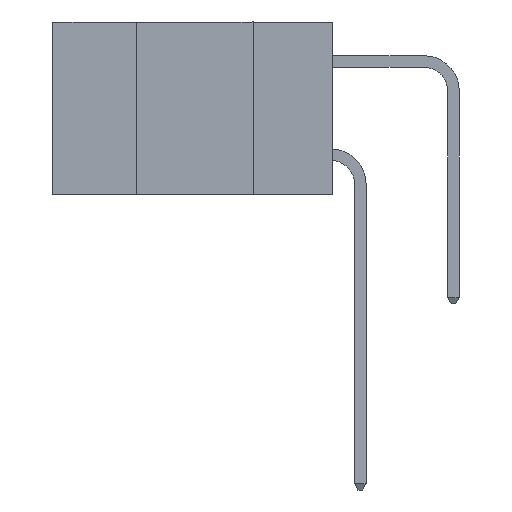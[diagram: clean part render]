
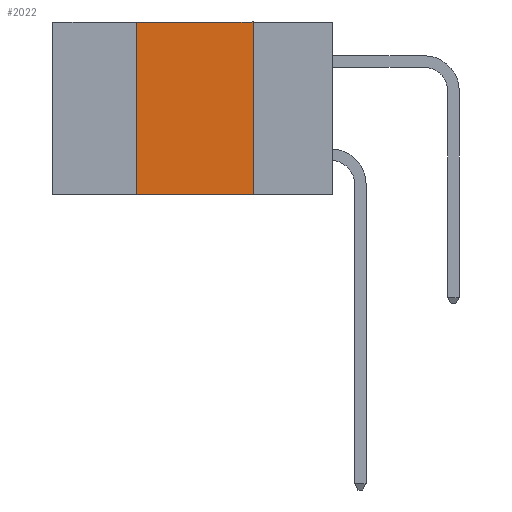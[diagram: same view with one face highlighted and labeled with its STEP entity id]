
A CAD part, left-side view. The second image highlights one B-rep face of the part: STEP entity #2022.
In plain terms, the highlighted planar face has unit normal (-1, 0, 0).
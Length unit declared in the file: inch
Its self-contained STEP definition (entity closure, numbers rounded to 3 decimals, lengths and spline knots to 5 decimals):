
#103 = EDGE_CURVE ( 'NONE', #596, #6846, #8828, .T. ) ;
#596 = VERTEX_POINT ( 'NONE', #9519 ) ;
#1050 = LINE ( 'NONE', #5411, #5491 ) ;
#1703 = CARTESIAN_POINT ( 'NONE',  ( 0., 0.6, -0.37 ) ) ;
#2022 = ADVANCED_FACE ( 'NONE', ( #6576 ), #9445, .F. ) ;
#2457 = ORIENTED_EDGE ( 'NONE', *, *, #3716, .T. ) ;
#2531 = EDGE_CURVE ( 'NONE', #5552, #596, #1050, .T. ) ;
#2717 = VERTEX_POINT ( 'NONE', #7918 ) ;
#3564 = DIRECTION ( 'NONE',  ( 0., -1., 0. ) ) ;
#3716 = EDGE_CURVE ( 'NONE', #5552, #2717, #4351, .T. ) ;
#4351 = LINE ( 'NONE', #1703, #8158 ) ;
#5157 = AXIS2_PLACEMENT_3D ( 'NONE', #9506, #9406, #9393 ) ;
#5411 = CARTESIAN_POINT ( 'NONE',  ( 0., 0.42, -0.37 ) ) ;
#5452 = DIRECTION ( 'NONE',  ( 0., 0., 1. ) ) ;
#5491 = VECTOR ( 'NONE', #5452, 39.37008 ) ;
#5552 = VERTEX_POINT ( 'NONE', #6528 ) ;
#5959 = VECTOR ( 'NONE', #6719, 39.37008 ) ;
#5965 = CARTESIAN_POINT ( 'NONE',  ( 0., 0.17, -0.37 ) ) ;
#6528 = CARTESIAN_POINT ( 'NONE',  ( 0., 0.42, -0.37 ) ) ;
#6547 = ORIENTED_EDGE ( 'NONE', *, *, #2531, .F. ) ;
#6576 = FACE_OUTER_BOUND ( 'NONE', #7148, .T. ) ;
#6719 = DIRECTION ( 'NONE',  ( 0., 0., -1. ) ) ;
#6826 = VECTOR ( 'NONE', #3564, 39.37008 ) ;
#6846 = VERTEX_POINT ( 'NONE', #9738 ) ;
#7148 = EDGE_LOOP ( 'NONE', ( #9045, #8975, #6547, #2457 ) ) ;
#7631 = CARTESIAN_POINT ( 'NONE',  ( 0., 0.6, 0. ) ) ;
#7714 = LINE ( 'NONE', #5965, #5959 ) ;
#7918 = CARTESIAN_POINT ( 'NONE',  ( 0., 0.17, -0.37 ) ) ;
#8158 = VECTOR ( 'NONE', #8879, 39.37008 ) ;
#8828 = LINE ( 'NONE', #7631, #6826 ) ;
#8879 = DIRECTION ( 'NONE',  ( 0., -1., 0. ) ) ;
#8975 = ORIENTED_EDGE ( 'NONE', *, *, #103, .F. ) ;
#9045 = ORIENTED_EDGE ( 'NONE', *, *, #9551, .F. ) ;
#9393 = DIRECTION ( 'NONE',  ( 0., 0., -1. ) ) ;
#9406 = DIRECTION ( 'NONE',  ( 1., 0., 0. ) ) ;
#9445 = PLANE ( 'NONE',  #5157 ) ;
#9506 = CARTESIAN_POINT ( 'NONE',  ( 0., 0.6, 0. ) ) ;
#9519 = CARTESIAN_POINT ( 'NONE',  ( 0., 0.42, 0. ) ) ;
#9551 = EDGE_CURVE ( 'NONE', #6846, #2717, #7714, .T. ) ;
#9738 = CARTESIAN_POINT ( 'NONE',  ( 0., 0.17, 0. ) ) ;
